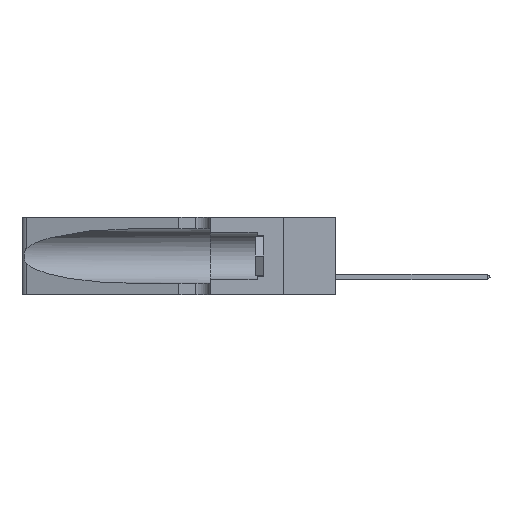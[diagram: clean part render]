
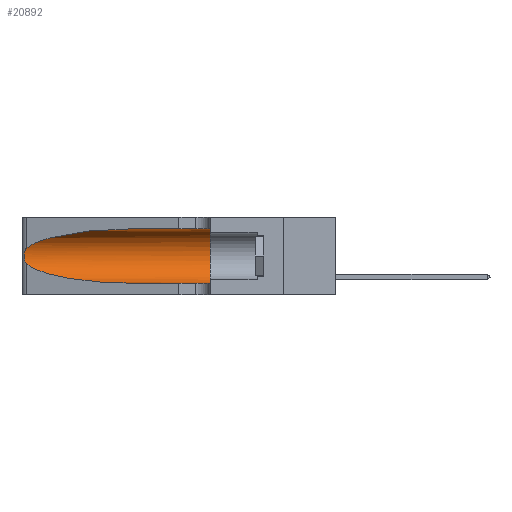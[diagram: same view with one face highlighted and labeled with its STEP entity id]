
A CAD part, left-side view. The second image highlights one B-rep face of the part: STEP entity #20892.
In plain terms, the highlighted cylindrical face has radius 3.308 mm (diameter 6.617 mm), a partial arc.
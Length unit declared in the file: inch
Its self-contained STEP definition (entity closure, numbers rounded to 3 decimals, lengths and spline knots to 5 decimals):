
#395 = VERTEX_POINT ( 'NONE', #1537 ) ;
#405 = CARTESIAN_POINT ( 'NONE',  ( 0.25487, 1.22718, 0.22369 ) ) ;
#669 = CARTESIAN_POINT ( 'NONE',  ( 0.2373, 1.15595, 0.28018 ) ) ;
#1068 = DIRECTION ( 'NONE',  ( 0., -1., 0. ) ) ;
#1307 = VERTEX_POINT ( 'NONE', #23263 ) ;
#1537 = CARTESIAN_POINT ( 'NONE',  ( 0.25487, 1.22718, 0.14631 ) ) ;
#1663 = ORIENTED_EDGE ( 'NONE', *, *, #24715, .T. ) ;
#2089 = CARTESIAN_POINT ( 'NONE',  ( 0.25487, 1.22718, 0.14631 ) ) ;
#2458 = EDGE_CURVE ( 'NONE', #1307, #9562, #3725, .T. ) ;
#2462 = CARTESIAN_POINT ( 'NONE',  ( 0.26018, 1.23835, 0.19895 ) ) ;
#2712 = CARTESIAN_POINT ( 'NONE',  ( 0.25639, 1.23186, 0.15144 ) ) ;
#3021 = ORIENTED_EDGE ( 'NONE', *, *, #12976, .T. ) ;
#3026 = ORIENTED_EDGE ( 'NONE', *, *, #6768, .F. ) ;
#3327 = CARTESIAN_POINT ( 'NONE',  ( 0.1305, 0.35, 0.31525 ) ) ;
#3725 =( BOUNDED_CURVE ( )  B_SPLINE_CURVE ( 3, ( #17184, #13456, #669, #18169 ),
 .UNSPECIFIED., .F., .T. ) 
 B_SPLINE_CURVE_WITH_KNOTS ( ( 4, 4 ),
 ( 1.5708, 2.84003 ),
 .UNSPECIFIED. ) 
 CURVE ( )  GEOMETRIC_REPRESENTATION_ITEM ( )  RATIONAL_B_SPLINE_CURVE ( ( 1., 0.87, 0.87, 1. ) ) 
 REPRESENTATION_ITEM ( '' )  );
#4121 = LINE ( 'NONE', #8549, #17214 ) ;
#5204 = VECTOR ( 'NONE', #10449, 39.37008 ) ;
#6083 = CARTESIAN_POINT ( 'NONE',  ( 0.1305, 1.61858, 0.185 ) ) ;
#6763 = CARTESIAN_POINT ( 'NONE',  ( 0.1305, 0.35, 0.185 ) ) ;
#6768 = EDGE_CURVE ( 'NONE', #1307, #11953, #24633, .T. ) ;
#8018 = AXIS2_PLACEMENT_3D ( 'NONE', #6763, #8710, #24224 ) ;
#8252 = CARTESIAN_POINT ( 'NONE',  ( 0.1305, 0.72297, 0.05475 ) ) ;
#8549 = CARTESIAN_POINT ( 'NONE',  ( 0.1305, 1.61858, 0.05475 ) ) ;
#8682 = FACE_OUTER_BOUND ( 'NONE', #16299, .T. ) ;
#8710 = DIRECTION ( 'NONE',  ( 0., 1., 0. ) ) ;
#9562 = VERTEX_POINT ( 'NONE', #24761 ) ;
#10449 = DIRECTION ( 'NONE',  ( 0., -1., 0. ) ) ;
#10513 = EDGE_CURVE ( 'NONE', #23517, #24145, #4121, .T. ) ;
#10711 = CARTESIAN_POINT ( 'NONE',  ( 0.25555, 1.22993, 0.14849 ) ) ;
#11264 =( BOUNDED_CURVE ( )  B_SPLINE_CURVE ( 3, ( #2089, #15770, #23437, #19467 ),
 .UNSPECIFIED., .F., .T. ) 
 B_SPLINE_CURVE_WITH_KNOTS ( ( 4, 4 ),
 ( 3.44316, 4.71239 ),
 .UNSPECIFIED. ) 
 CURVE ( )  GEOMETRIC_REPRESENTATION_ITEM ( )  RATIONAL_B_SPLINE_CURVE ( ( 1., 0.87, 0.87, 1. ) ) 
 REPRESENTATION_ITEM ( '' )  );
#11953 = VERTEX_POINT ( 'NONE', #3327 ) ;
#12053 = CARTESIAN_POINT ( 'NONE',  ( 0.26075, 1.23896, 0.19203 ) ) ;
#12220 = CARTESIAN_POINT ( 'NONE',  ( 0.26017, 1.23833, 0.17102 ) ) ;
#12311 = CARTESIAN_POINT ( 'NONE',  ( 0.25789, 1.23486, 0.15765 ) ) ;
#12478 = B_SPLINE_CURVE_WITH_KNOTS ( 'NONE', 3,
 ( #405, #23823, #21744, #14037, #19745, #2462, #12053, #18074, #12220, #23912, #12311, #2712, #10711, #16377 ),
 .UNSPECIFIED., .F., .F.,
 ( 4, 2, 2, 2, 2, 2, 4 ),
 ( 0., 0.00027, 0.00053, 0.00107, 0.0016, 0.00187, 0.00214 ),
 .UNSPECIFIED. ) ;
#12976 = EDGE_CURVE ( 'NONE', #9562, #395, #12478, .T. ) ;
#13063 = AXIS2_PLACEMENT_3D ( 'NONE', #6083, #14425, #15679 ) ;
#13260 = CYLINDRICAL_SURFACE ( 'NONE', #13063, 0.13025 ) ;
#13456 = CARTESIAN_POINT ( 'NONE',  ( 0.18966, 0.96281, 0.31525 ) ) ;
#14037 = CARTESIAN_POINT ( 'NONE',  ( 0.25787, 1.23484, 0.2124 ) ) ;
#14425 = DIRECTION ( 'NONE',  ( 0., -1., 0. ) ) ;
#15642 = CARTESIAN_POINT ( 'NONE',  ( 0.1305, 0.35, 0.05475 ) ) ;
#15654 = CIRCLE ( 'NONE', #8018, 0.13025 ) ;
#15679 = DIRECTION ( 'NONE',  ( 0., 0., -1. ) ) ;
#15770 = CARTESIAN_POINT ( 'NONE',  ( 0.2373, 1.15595, 0.08982 ) ) ;
#16299 = EDGE_LOOP ( 'NONE', ( #24298, #3021, #1663, #18268, #23424, #3026 ) ) ;
#16360 = CARTESIAN_POINT ( 'NONE',  ( 0.1305, 1.61858, 0.31525 ) ) ;
#16377 = CARTESIAN_POINT ( 'NONE',  ( 0.25487, 1.22718, 0.14631 ) ) ;
#17184 = CARTESIAN_POINT ( 'NONE',  ( 0.1305, 0.72297, 0.31525 ) ) ;
#17214 = VECTOR ( 'NONE', #1068, 39.37008 ) ;
#18074 = CARTESIAN_POINT ( 'NONE',  ( 0.26075, 1.23896, 0.178 ) ) ;
#18169 = CARTESIAN_POINT ( 'NONE',  ( 0.25487, 1.22718, 0.22369 ) ) ;
#18268 = ORIENTED_EDGE ( 'NONE', *, *, #10513, .T. ) ;
#19467 = CARTESIAN_POINT ( 'NONE',  ( 0.1305, 0.72297, 0.05475 ) ) ;
#19745 = CARTESIAN_POINT ( 'NONE',  ( 0.25854, 1.2359, 0.20912 ) ) ;
#20892 = ADVANCED_FACE ( 'NONE', ( #8682 ), #13260, .F. ) ;
#21744 = CARTESIAN_POINT ( 'NONE',  ( 0.25639, 1.23184, 0.21858 ) ) ;
#21755 = EDGE_CURVE ( 'NONE', #11953, #24145, #15654, .T. ) ;
#23263 = CARTESIAN_POINT ( 'NONE',  ( 0.1305, 0.72297, 0.31525 ) ) ;
#23424 = ORIENTED_EDGE ( 'NONE', *, *, #21755, .F. ) ;
#23437 = CARTESIAN_POINT ( 'NONE',  ( 0.18966, 0.96281, 0.05475 ) ) ;
#23517 = VERTEX_POINT ( 'NONE', #8252 ) ;
#23823 = CARTESIAN_POINT ( 'NONE',  ( 0.25555, 1.22994, 0.2215 ) ) ;
#23912 = CARTESIAN_POINT ( 'NONE',  ( 0.25856, 1.23593, 0.16098 ) ) ;
#24145 = VERTEX_POINT ( 'NONE', #15642 ) ;
#24224 = DIRECTION ( 'NONE',  ( 0., 0., 1. ) ) ;
#24298 = ORIENTED_EDGE ( 'NONE', *, *, #2458, .T. ) ;
#24633 = LINE ( 'NONE', #16360, #5204 ) ;
#24715 = EDGE_CURVE ( 'NONE', #395, #23517, #11264, .T. ) ;
#24761 = CARTESIAN_POINT ( 'NONE',  ( 0.25487, 1.22718, 0.22369 ) ) ;
